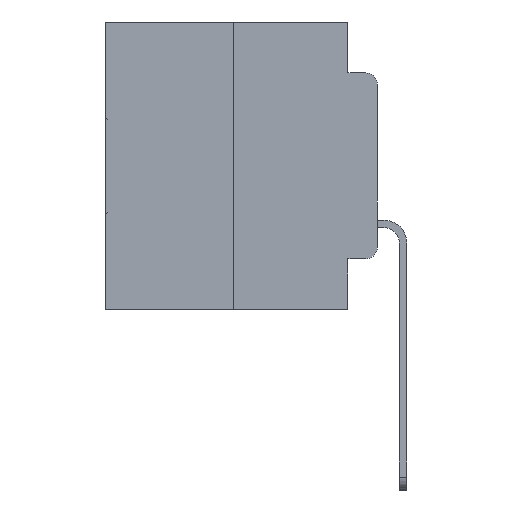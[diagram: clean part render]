
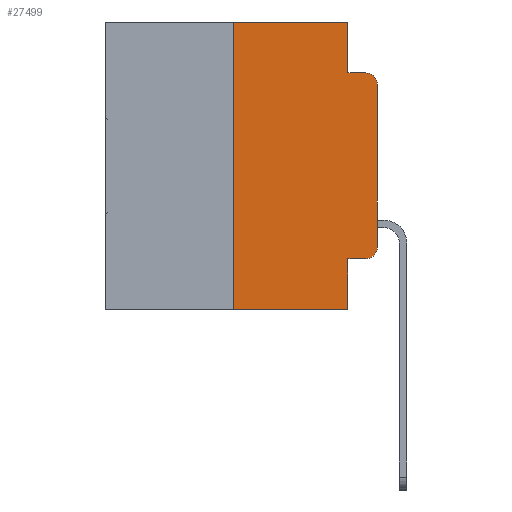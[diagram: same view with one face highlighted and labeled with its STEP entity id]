
A CAD part, left-side view. The second image highlights one B-rep face of the part: STEP entity #27499.
In plain terms, the highlighted planar face has unit normal (-1, 0, 0).
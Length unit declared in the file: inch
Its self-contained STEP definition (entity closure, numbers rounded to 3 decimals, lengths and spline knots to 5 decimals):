
#1134 = VERTEX_POINT ( 'NONE', #17452 ) ;
#1397 = EDGE_LOOP ( 'NONE', ( #15491, #16929, #24512, #24181, #10778, #25258, #29371, #29053, #25809, #27605 ) ) ;
#1773 = VERTEX_POINT ( 'NONE', #17881 ) ;
#2897 = VECTOR ( 'NONE', #23498, 39.37008 ) ;
#3137 = DIRECTION ( 'NONE',  ( -1., 0., 0. ) ) ;
#4584 = CARTESIAN_POINT ( 'NONE',  ( 0., 0.051, -0.4115 ) ) ;
#4853 = AXIS2_PLACEMENT_3D ( 'NONE', #6101, #22438, #8559 ) ;
#4882 = EDGE_CURVE ( 'NONE', #11453, #15174, #8272, .T. ) ;
#5676 = VECTOR ( 'NONE', #21205, 39.37008 ) ;
#6101 = CARTESIAN_POINT ( 'NONE',  ( 0., 0.02, -0.3915 ) ) ;
#6132 = LINE ( 'NONE', #22976, #13064 ) ;
#6890 = CIRCLE ( 'NONE', #4853, 0.02 ) ;
#7055 = VERTEX_POINT ( 'NONE', #21540 ) ;
#7193 = DIRECTION ( 'NONE',  ( 0., 0., 1. ) ) ;
#7663 = CIRCLE ( 'NONE', #10638, 0.02 ) ;
#8106 = VECTOR ( 'NONE', #30476, 39.37008 ) ;
#8272 = LINE ( 'NONE', #17676, #19888 ) ;
#8380 = VECTOR ( 'NONE', #7193, 39.37008 ) ;
#8559 = DIRECTION ( 'NONE',  ( 0., 0., -1. ) ) ;
#9126 = EDGE_CURVE ( 'NONE', #21986, #19203, #6132, .T. ) ;
#9585 = LINE ( 'NONE', #4584, #2897 ) ;
#9697 = EDGE_CURVE ( 'NONE', #7055, #21986, #6890, .T. ) ;
#9804 = LINE ( 'NONE', #14272, #5676 ) ;
#10050 = EDGE_CURVE ( 'NONE', #15174, #12226, #9804, .T. ) ;
#10588 = CARTESIAN_POINT ( 'NONE',  ( 0., 0., -0.3915 ) ) ;
#10638 = AXIS2_PLACEMENT_3D ( 'NONE', #17514, #3137, #19877 ) ;
#10778 = ORIENTED_EDGE ( 'NONE', *, *, #4882, .F. ) ;
#11453 = VERTEX_POINT ( 'NONE', #12022 ) ;
#11676 = CARTESIAN_POINT ( 'NONE',  ( 0., 0.051, -0.0885 ) ) ;
#11946 = LINE ( 'NONE', #18689, #29700 ) ;
#12022 = CARTESIAN_POINT ( 'NONE',  ( 0., 0.25, 0. ) ) ;
#12226 = VERTEX_POINT ( 'NONE', #15046 ) ;
#12572 = EDGE_CURVE ( 'NONE', #12226, #1773, #18948, .T. ) ;
#13064 = VECTOR ( 'NONE', #20557, 39.37008 ) ;
#13376 = CARTESIAN_POINT ( 'NONE',  ( 0., 0.051, 0. ) ) ;
#14044 = DIRECTION ( 'NONE',  ( 1., 0., 0. ) ) ;
#14178 = VECTOR ( 'NONE', #25546, 39.37008 ) ;
#14272 = CARTESIAN_POINT ( 'NONE',  ( 0., 0.051, 0. ) ) ;
#14328 = CARTESIAN_POINT ( 'NONE',  ( 0., 0.473, -0.5 ) ) ;
#15046 = CARTESIAN_POINT ( 'NONE',  ( 0., 0.051, -0.0885 ) ) ;
#15174 = VERTEX_POINT ( 'NONE', #13376 ) ;
#15491 = ORIENTED_EDGE ( 'NONE', *, *, #9126, .T. ) ;
#16929 = ORIENTED_EDGE ( 'NONE', *, *, #25362, .T. ) ;
#17452 = CARTESIAN_POINT ( 'NONE',  ( 0., 0.25, -0.5 ) ) ;
#17514 = CARTESIAN_POINT ( 'NONE',  ( 0., 0.02, -0.1085 ) ) ;
#17676 = CARTESIAN_POINT ( 'NONE',  ( 0., 0.473, 0. ) ) ;
#17881 = CARTESIAN_POINT ( 'NONE',  ( 0., 0.02, -0.0885 ) ) ;
#18689 = CARTESIAN_POINT ( 'NONE',  ( 0., 0.051, 0. ) ) ;
#18780 = CARTESIAN_POINT ( 'NONE',  ( 0., 0.25, 0. ) ) ;
#18948 = LINE ( 'NONE', #11676, #14178 ) ;
#19051 = EDGE_CURVE ( 'NONE', #1134, #23890, #21164, .T. ) ;
#19057 = VERTEX_POINT ( 'NONE', #28191 ) ;
#19076 = AXIS2_PLACEMENT_3D ( 'NONE', #27925, #14044, #30204 ) ;
#19203 = VERTEX_POINT ( 'NONE', #23949 ) ;
#19688 = EDGE_CURVE ( 'NONE', #19057, #23890, #11946, .T. ) ;
#19859 = EDGE_CURVE ( 'NONE', #1134, #11453, #26086, .T. ) ;
#19877 = DIRECTION ( 'NONE',  ( 0., 0., -1. ) ) ;
#19888 = VECTOR ( 'NONE', #26963, 39.37008 ) ;
#20557 = DIRECTION ( 'NONE',  ( 0., 0., 1. ) ) ;
#21019 = DIRECTION ( 'NONE',  ( 0., 0., -1. ) ) ;
#21164 = LINE ( 'NONE', #14328, #8106 ) ;
#21205 = DIRECTION ( 'NONE',  ( 0., 0., -1. ) ) ;
#21540 = CARTESIAN_POINT ( 'NONE',  ( 0., 0.02, -0.4115 ) ) ;
#21986 = VERTEX_POINT ( 'NONE', #10588 ) ;
#22438 = DIRECTION ( 'NONE',  ( -1., 0., 0. ) ) ;
#22976 = CARTESIAN_POINT ( 'NONE',  ( 0., 0., 0. ) ) ;
#23498 = DIRECTION ( 'NONE',  ( 0., -1., 0. ) ) ;
#23890 = VERTEX_POINT ( 'NONE', #25878 ) ;
#23949 = CARTESIAN_POINT ( 'NONE',  ( 0., 0., -0.1085 ) ) ;
#24181 = ORIENTED_EDGE ( 'NONE', *, *, #10050, .F. ) ;
#24512 = ORIENTED_EDGE ( 'NONE', *, *, #12572, .F. ) ;
#25258 = ORIENTED_EDGE ( 'NONE', *, *, #19859, .F. ) ;
#25362 = EDGE_CURVE ( 'NONE', #19203, #1773, #7663, .T. ) ;
#25546 = DIRECTION ( 'NONE',  ( 0., -1., 0. ) ) ;
#25586 = PLANE ( 'NONE',  #19076 ) ;
#25809 = ORIENTED_EDGE ( 'NONE', *, *, #27544, .T. ) ;
#25878 = CARTESIAN_POINT ( 'NONE',  ( 0., 0.051, -0.5 ) ) ;
#26086 = LINE ( 'NONE', #18780, #8380 ) ;
#26963 = DIRECTION ( 'NONE',  ( 0., -1., 0. ) ) ;
#27499 = ADVANCED_FACE ( 'NONE', ( #30166 ), #25586, .F. ) ;
#27544 = EDGE_CURVE ( 'NONE', #19057, #7055, #9585, .T. ) ;
#27605 = ORIENTED_EDGE ( 'NONE', *, *, #9697, .T. ) ;
#27925 = CARTESIAN_POINT ( 'NONE',  ( 0., 0.473, 0. ) ) ;
#28191 = CARTESIAN_POINT ( 'NONE',  ( 0., 0.051, -0.4115 ) ) ;
#29053 = ORIENTED_EDGE ( 'NONE', *, *, #19688, .F. ) ;
#29371 = ORIENTED_EDGE ( 'NONE', *, *, #19051, .T. ) ;
#29700 = VECTOR ( 'NONE', #21019, 39.37008 ) ;
#30166 = FACE_OUTER_BOUND ( 'NONE', #1397, .T. ) ;
#30204 = DIRECTION ( 'NONE',  ( 0., 0., -1. ) ) ;
#30476 = DIRECTION ( 'NONE',  ( 0., -1., 0. ) ) ;
